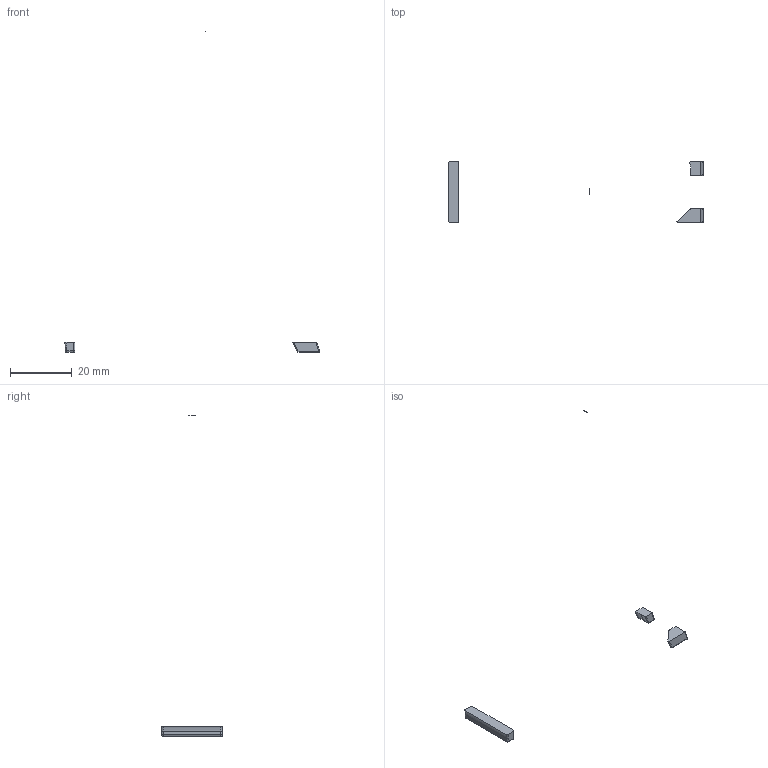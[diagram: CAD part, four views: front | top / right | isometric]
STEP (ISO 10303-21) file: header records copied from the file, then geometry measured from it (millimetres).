
FILE_DESCRIPTION(/* description */ (''),/* implementation_level */ '2;1');
FILE_NAME(/* name */ 'parts removed.stp',/* time_stamp */ '2019-10-25T14:37:38+03:00',/* author */ (''),/* organization */ (''),/* preprocessor_version */ 'ST-DEVELOPER v15.2',/* originating_system */ 'Autodesk Translator Framework v2.0.0.5431',/* authorisation */ '');
FILE_SCHEMA (('AUTOMOTIVE_DESIGN { 1 0 10303 214 3 1 1 }'));
Length unit declared in the file: centimetre
Products named in the file (1): WOKING PARTS
Bounding box: 82.48 x 19.62 x 103.61 mm (x, y, z)
Volume: 329 mm3; surface area: 461.3 mm2
Topology: 4 solids, 4 shells, 62 faces, 124 edges, 70 vertices
Faces by surface type: cylinder 27, plane 20, sphere 11, bspline 2, torus 2
Entity records: 1652 total; most frequent: CARTESIAN_POINT 313, DIRECTION 303, ORIENTED_EDGE 248, EDGE_CURVE 124, AXIS2_PLACEMENT_3D 120, VERTEX_POINT 70, LINE 63, VECTOR 63
